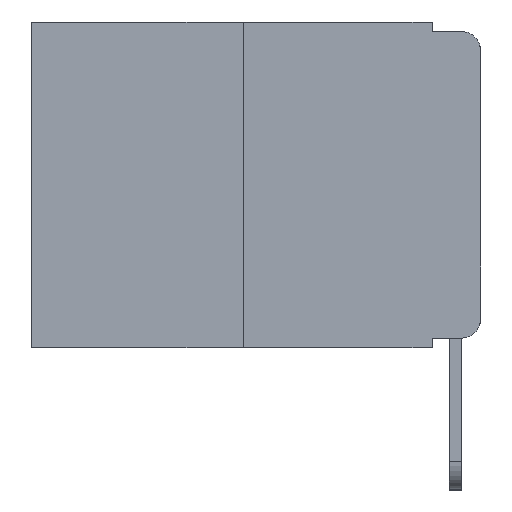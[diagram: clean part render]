
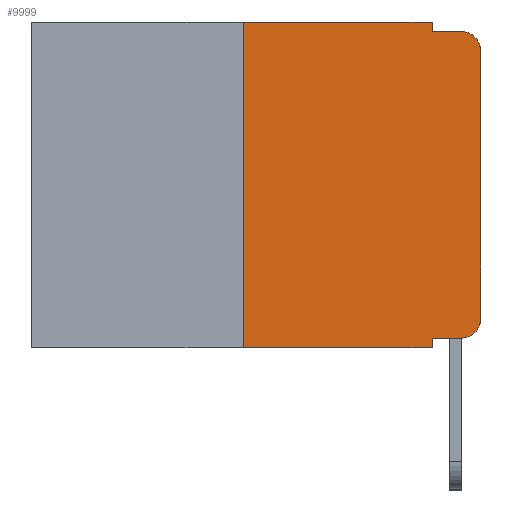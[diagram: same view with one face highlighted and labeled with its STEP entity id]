
A CAD part, left-side view. The second image highlights one B-rep face of the part: STEP entity #9999.
In plain terms, the highlighted planar face has unit normal (-1, 0, 0).
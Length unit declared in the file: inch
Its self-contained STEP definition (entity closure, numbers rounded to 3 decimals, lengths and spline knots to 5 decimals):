
#90 = ORIENTED_EDGE ( 'NONE', *, *, #3019, .F. ) ;
#130 = ORIENTED_EDGE ( 'NONE', *, *, #14162, .T. ) ;
#148 = DIRECTION ( 'NONE',  ( 0., -1., 0. ) ) ;
#230 = VECTOR ( 'NONE', #14167, 39.37008 ) ;
#356 = LINE ( 'NONE', #815, #11676 ) ;
#541 = CIRCLE ( 'NONE', #5673, 0.02 ) ;
#815 = CARTESIAN_POINT ( 'NONE',  ( 0., 0.25, 0. ) ) ;
#861 = EDGE_CURVE ( 'NONE', #4018, #6109, #12659, .T. ) ;
#1010 = CARTESIAN_POINT ( 'NONE',  ( 0., 0.02, -0.333 ) ) ;
#1128 = EDGE_CURVE ( 'NONE', #11739, #7596, #12273, .T. ) ;
#1269 = DIRECTION ( 'NONE',  ( 0., -1., 0. ) ) ;
#1312 = ORIENTED_EDGE ( 'NONE', *, *, #861, .T. ) ;
#1604 = DIRECTION ( 'NONE',  ( -1., 0., 0. ) ) ;
#1757 = CARTESIAN_POINT ( 'NONE',  ( 0., 0.25, -0.343 ) ) ;
#1917 = VERTEX_POINT ( 'NONE', #1944 ) ;
#1944 = CARTESIAN_POINT ( 'NONE',  ( 0., 0., -0.03 ) ) ;
#2261 = ORIENTED_EDGE ( 'NONE', *, *, #11348, .F. ) ;
#2287 = VERTEX_POINT ( 'NONE', #10692 ) ;
#2513 = LINE ( 'NONE', #3196, #7083 ) ;
#2806 = VECTOR ( 'NONE', #11699, 39.37008 ) ;
#3019 = EDGE_CURVE ( 'NONE', #4018, #7596, #11624, .T. ) ;
#3196 = CARTESIAN_POINT ( 'NONE',  ( 0., 0.051, 0. ) ) ;
#3861 = AXIS2_PLACEMENT_3D ( 'NONE', #4966, #1604, #3976 ) ;
#3944 = CARTESIAN_POINT ( 'NONE',  ( 0., 0.473, -0.343 ) ) ;
#3976 = DIRECTION ( 'NONE',  ( 0., 0., -1. ) ) ;
#3982 = VECTOR ( 'NONE', #1269, 39.37008 ) ;
#4018 = VERTEX_POINT ( 'NONE', #12232 ) ;
#4547 = VERTEX_POINT ( 'NONE', #7007 ) ;
#4600 = VECTOR ( 'NONE', #14645, 39.37008 ) ;
#4660 = VERTEX_POINT ( 'NONE', #8520 ) ;
#4966 = CARTESIAN_POINT ( 'NONE',  ( 0., 0.02, -0.03 ) ) ;
#5392 = ORIENTED_EDGE ( 'NONE', *, *, #11450, .F. ) ;
#5673 = AXIS2_PLACEMENT_3D ( 'NONE', #11840, #7477, #13205 ) ;
#5886 = VECTOR ( 'NONE', #148, 39.37008 ) ;
#5935 = CARTESIAN_POINT ( 'NONE',  ( 0., 0., 0. ) ) ;
#5986 = EDGE_CURVE ( 'NONE', #6109, #2287, #541, .T. ) ;
#6109 = VERTEX_POINT ( 'NONE', #1010 ) ;
#6190 = DIRECTION ( 'NONE',  ( 1., 0., 0. ) ) ;
#6608 = FACE_OUTER_BOUND ( 'NONE', #6971, .T. ) ;
#6971 = EDGE_LOOP ( 'NONE', ( #130, #10370, #7978, #2261, #5392, #9833, #11724, #90, #1312, #10717 ) ) ;
#7007 = CARTESIAN_POINT ( 'NONE',  ( 0., 0.02, -0.01 ) ) ;
#7060 = VERTEX_POINT ( 'NONE', #9081 ) ;
#7083 = VECTOR ( 'NONE', #9954, 39.37008 ) ;
#7099 = CIRCLE ( 'NONE', #3861, 0.02 ) ;
#7300 = AXIS2_PLACEMENT_3D ( 'NONE', #9696, #6190, #9737 ) ;
#7423 = EDGE_CURVE ( 'NONE', #11739, #4660, #356, .T. ) ;
#7477 = DIRECTION ( 'NONE',  ( -1., 0., 0. ) ) ;
#7596 = VERTEX_POINT ( 'NONE', #13397 ) ;
#7757 = CARTESIAN_POINT ( 'NONE',  ( 0., 0.473, 0. ) ) ;
#7978 = ORIENTED_EDGE ( 'NONE', *, *, #13870, .F. ) ;
#8520 = CARTESIAN_POINT ( 'NONE',  ( 0., 0.25, 0. ) ) ;
#8601 = PLANE ( 'NONE',  #7300 ) ;
#8878 = CARTESIAN_POINT ( 'NONE',  ( 0., 0.051, -0.01 ) ) ;
#8976 = CARTESIAN_POINT ( 'NONE',  ( 0., 0.051, -0.333 ) ) ;
#9081 = CARTESIAN_POINT ( 'NONE',  ( 0., 0.051, 0. ) ) ;
#9696 = CARTESIAN_POINT ( 'NONE',  ( 0., 0.473, 0. ) ) ;
#9737 = DIRECTION ( 'NONE',  ( 0., 0., -1. ) ) ;
#9833 = ORIENTED_EDGE ( 'NONE', *, *, #7423, .F. ) ;
#9954 = DIRECTION ( 'NONE',  ( 0., 0., -1. ) ) ;
#9999 = ADVANCED_FACE ( 'NONE', ( #6608 ), #8601, .F. ) ;
#10370 = ORIENTED_EDGE ( 'NONE', *, *, #11750, .T. ) ;
#10404 = VECTOR ( 'NONE', #13745, 39.37008 ) ;
#10692 = CARTESIAN_POINT ( 'NONE',  ( 0., 0., -0.313 ) ) ;
#10717 = ORIENTED_EDGE ( 'NONE', *, *, #5986, .T. ) ;
#10894 = DIRECTION ( 'NONE',  ( 0., 0., 1. ) ) ;
#10995 = CARTESIAN_POINT ( 'NONE',  ( 0., 0.051, -0.01 ) ) ;
#11348 = EDGE_CURVE ( 'NONE', #7060, #14441, #2513, .T. ) ;
#11445 = CARTESIAN_POINT ( 'NONE',  ( 0., 0.051, 0. ) ) ;
#11450 = EDGE_CURVE ( 'NONE', #4660, #7060, #14185, .T. ) ;
#11624 = LINE ( 'NONE', #11445, #10404 ) ;
#11676 = VECTOR ( 'NONE', #10894, 39.37008 ) ;
#11699 = DIRECTION ( 'NONE',  ( 0., 0., 1. ) ) ;
#11724 = ORIENTED_EDGE ( 'NONE', *, *, #1128, .T. ) ;
#11739 = VERTEX_POINT ( 'NONE', #1757 ) ;
#11750 = EDGE_CURVE ( 'NONE', #1917, #4547, #7099, .T. ) ;
#11840 = CARTESIAN_POINT ( 'NONE',  ( 0., 0.02, -0.313 ) ) ;
#12232 = CARTESIAN_POINT ( 'NONE',  ( 0., 0.051, -0.333 ) ) ;
#12273 = LINE ( 'NONE', #3944, #230 ) ;
#12659 = LINE ( 'NONE', #8976, #3982 ) ;
#13205 = DIRECTION ( 'NONE',  ( 0., 0., -1. ) ) ;
#13397 = CARTESIAN_POINT ( 'NONE',  ( 0., 0.051, -0.343 ) ) ;
#13612 = LINE ( 'NONE', #8878, #4600 ) ;
#13745 = DIRECTION ( 'NONE',  ( 0., 0., -1. ) ) ;
#13870 = EDGE_CURVE ( 'NONE', #14441, #4547, #13612, .T. ) ;
#14120 = LINE ( 'NONE', #5935, #2806 ) ;
#14162 = EDGE_CURVE ( 'NONE', #2287, #1917, #14120, .T. ) ;
#14167 = DIRECTION ( 'NONE',  ( 0., -1., 0. ) ) ;
#14185 = LINE ( 'NONE', #7757, #5886 ) ;
#14441 = VERTEX_POINT ( 'NONE', #10995 ) ;
#14645 = DIRECTION ( 'NONE',  ( 0., -1., 0. ) ) ;
